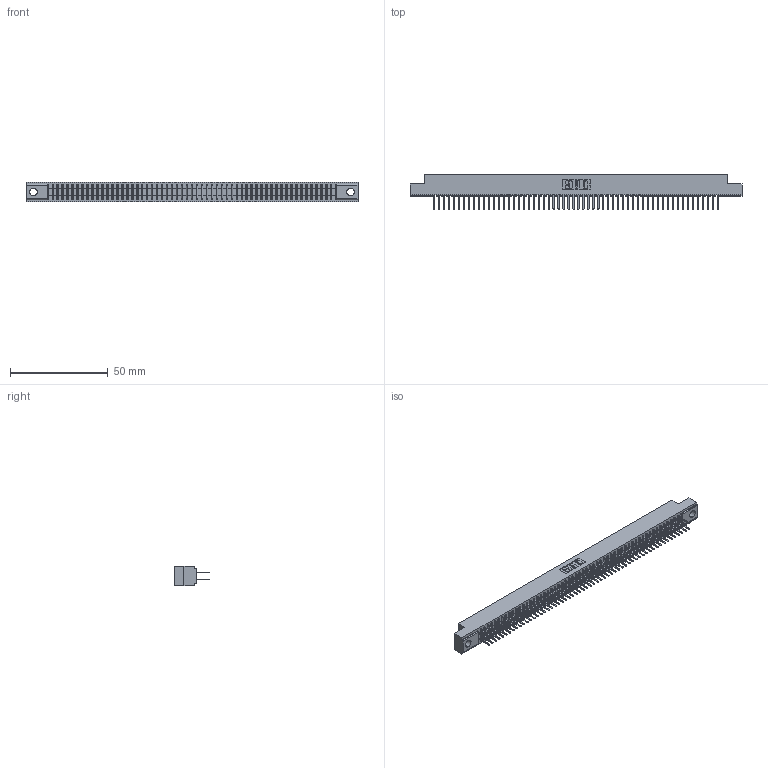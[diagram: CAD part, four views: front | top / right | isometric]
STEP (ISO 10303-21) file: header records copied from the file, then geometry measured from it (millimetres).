
FILE_DESCRIPTION (( 'STEP AP203' ), '1' );
FILE_NAME ('341-116-521-204.STEP', '2018-08-08T13:55:37', ( '' ), ( '' ), 'SwSTEP 2.0', 'SolidWorks 2016', '' );
FILE_SCHEMA (( 'CONFIG_CONTROL_DESIGN' ));
Length unit declared in the file: inch
Products named in the file (3): 341-292-001_341-292-121; 341-116-521-204; 341 Part_.156 (3.96) Dia Mounting Holes
Assembly tree (117 placements, depth 2):
  341-116-521-204
    341 Part_.156 (3.96) Dia Mounting Holes
    341-292-001_341-292-121  x116
Bounding box: 169.54 x 17.7 x 10.16 mm (x, y, z)
Volume: 12516.1 mm3; surface area: 23120.1 mm2
Topology: 117 solids, 117 shells, 7786 faces, 22566 edges, 14614 vertices
Faces by surface type: plane 4722, cylinder 2832, sphere 118, torus 114
Entity records: 68479 total; most frequent: CARTESIAN_POINT 11388, ORIENTED_EDGE 11316, DIRECTION 11032, EDGE_CURVE 5658, LINE 4596, VECTOR 4596, VERTEX_POINT 3574, AXIS2_PLACEMENT_3D 3218
